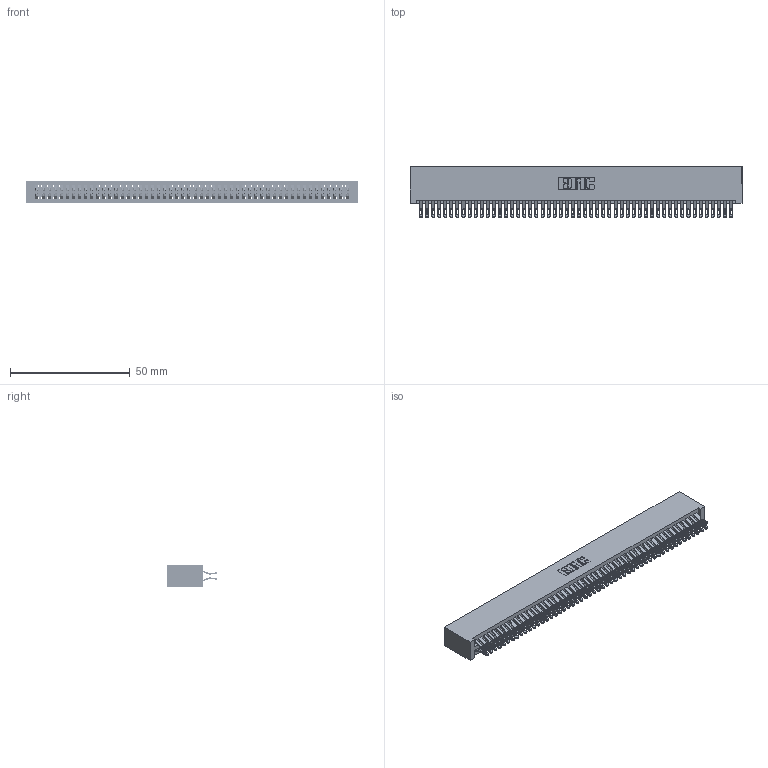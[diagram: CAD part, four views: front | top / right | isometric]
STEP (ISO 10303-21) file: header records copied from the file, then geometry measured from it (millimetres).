
FILE_DESCRIPTION (( 'STEP AP203' ), '1' );
FILE_NAME ('395-104-555-201.STEP', '2018-11-30T13:49:21', ( '' ), ( '' ), 'SwSTEP 2.0', 'SolidWorks 2016', '' );
FILE_SCHEMA (( 'CONFIG_CONTROL_DESIGN' ));
Length unit declared in the file: inch
Products named in the file (3): 345 Part_No Mounting Lugs; 345-292-001_555 Tail; 395-104-555-201
Assembly tree (105 placements, depth 2):
  395-104-555-201
    345 Part_No Mounting Lugs
    345-292-001_555 Tail  x104
Bounding box: 138.68 x 21.13 x 9.4 mm (x, y, z)
Volume: 14482.3 mm3; surface area: 22953.4 mm2
Topology: 105 solids, 105 shells, 5942 faces, 18725 edges, 12482 vertices
Faces by surface type: plane 3300, cylinder 2642
Entity records: 39503 total; most frequent: CARTESIAN_POINT 6646, ORIENTED_EDGE 6550, DIRECTION 5811, EDGE_CURVE 3275, VECTOR 2923, LINE 2923, VERTEX_POINT 2182, AXIS2_PLACEMENT_3D 1444
